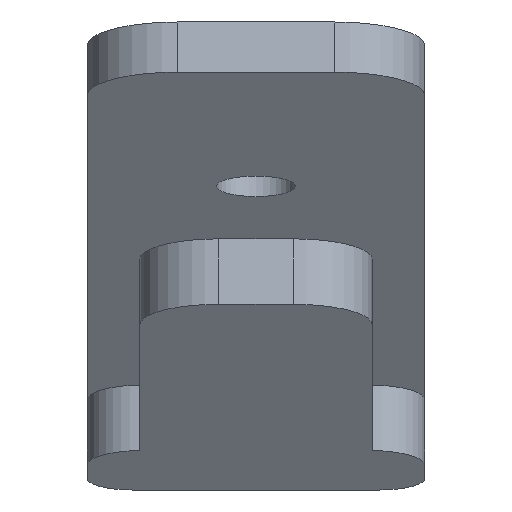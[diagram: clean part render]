
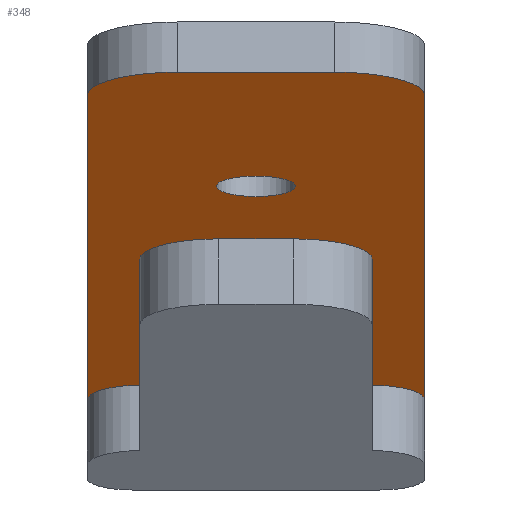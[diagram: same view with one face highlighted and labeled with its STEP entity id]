
A CAD part, left-side view. The second image highlights one B-rep face of the part: STEP entity #348.
In plain terms, the highlighted planar face has unit normal (-0.259, 0, -0.966).
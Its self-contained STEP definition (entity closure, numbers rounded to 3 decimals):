
#15=FACE_BOUND('',#48,.T.);
#17=PLANE('',#383);
#28=FACE_OUTER_BOUND('',#47,.T.);
#47=EDGE_LOOP('',(#240,#241,#242,#243,#244,#245,#246,#247,#248,#249,#250,
#251));
#48=EDGE_LOOP('',(#252));
#68=LINE('',#536,#101);
#69=LINE('',#540,#102);
#70=LINE('',#544,#103);
#71=LINE('',#548,#104);
#72=LINE('',#552,#105);
#73=LINE('',#556,#106);
#101=VECTOR('',#428,10.);
#102=VECTOR('',#431,10.);
#103=VECTOR('',#434,10.);
#104=VECTOR('',#437,10.);
#105=VECTOR('',#440,10.);
#106=VECTOR('',#443,10.);
#134=CIRCLE('',#382,1.75);
#135=CIRCLE('',#384,4.);
#136=CIRCLE('',#385,4.);
#137=CIRCLE('',#386,2.5);
#138=CIRCLE('',#387,3.5);
#139=CIRCLE('',#388,3.5);
#140=CIRCLE('',#389,2.5);
#152=VERTEX_POINT('',#530);
#153=VERTEX_POINT('',#534);
#154=VERTEX_POINT('',#535);
#155=VERTEX_POINT('',#537);
#156=VERTEX_POINT('',#539);
#157=VERTEX_POINT('',#541);
#158=VERTEX_POINT('',#543);
#159=VERTEX_POINT('',#545);
#160=VERTEX_POINT('',#547);
#161=VERTEX_POINT('',#549);
#162=VERTEX_POINT('',#551);
#163=VERTEX_POINT('',#553);
#164=VERTEX_POINT('',#555);
#187=EDGE_CURVE('',#152,#152,#134,.T.);
#188=EDGE_CURVE('',#153,#154,#68,.T.);
#189=EDGE_CURVE('',#154,#155,#135,.T.);
#190=EDGE_CURVE('',#155,#156,#69,.T.);
#191=EDGE_CURVE('',#156,#157,#136,.T.);
#192=EDGE_CURVE('',#157,#158,#70,.T.);
#193=EDGE_CURVE('',#159,#158,#137,.T.);
#194=EDGE_CURVE('',#160,#159,#71,.T.);
#195=EDGE_CURVE('',#161,#160,#138,.T.);
#196=EDGE_CURVE('',#162,#161,#72,.T.);
#197=EDGE_CURVE('',#163,#162,#139,.T.);
#198=EDGE_CURVE('',#164,#163,#73,.T.);
#199=EDGE_CURVE('',#153,#164,#140,.T.);
#240=ORIENTED_EDGE('',*,*,#188,.T.);
#241=ORIENTED_EDGE('',*,*,#189,.T.);
#242=ORIENTED_EDGE('',*,*,#190,.T.);
#243=ORIENTED_EDGE('',*,*,#191,.T.);
#244=ORIENTED_EDGE('',*,*,#192,.T.);
#245=ORIENTED_EDGE('',*,*,#193,.F.);
#246=ORIENTED_EDGE('',*,*,#194,.F.);
#247=ORIENTED_EDGE('',*,*,#195,.F.);
#248=ORIENTED_EDGE('',*,*,#196,.F.);
#249=ORIENTED_EDGE('',*,*,#197,.F.);
#250=ORIENTED_EDGE('',*,*,#198,.F.);
#251=ORIENTED_EDGE('',*,*,#199,.F.);
#252=ORIENTED_EDGE('',*,*,#187,.F.);
#348=ADVANCED_FACE('',(#28,#15),#17,.T.);
#382=AXIS2_PLACEMENT_3D('',#532,#424,#425);
#383=AXIS2_PLACEMENT_3D('',#533,#426,#427);
#384=AXIS2_PLACEMENT_3D('',#538,#429,#430);
#385=AXIS2_PLACEMENT_3D('',#542,#432,#433);
#386=AXIS2_PLACEMENT_3D('',#546,#435,#436);
#387=AXIS2_PLACEMENT_3D('',#550,#438,#439);
#388=AXIS2_PLACEMENT_3D('',#554,#441,#442);
#389=AXIS2_PLACEMENT_3D('',#557,#444,#445);
#424=DIRECTION('center_axis',(-0.259,0.,
-0.966));
#425=DIRECTION('ref_axis',(0.,-1.,0.));
#426=DIRECTION('center_axis',(-0.259,0.,
-0.966));
#427=DIRECTION('ref_axis',(0.,-1.,0.));
#428=DIRECTION('',(-0.966,0.,0.259));
#429=DIRECTION('center_axis',(-0.259,0.,
-0.966));
#430=DIRECTION('ref_axis',(0.,-1.,0.));
#431=DIRECTION('',(0.,1.,0.));
#432=DIRECTION('center_axis',(-0.259,0.,
-0.966));
#433=DIRECTION('ref_axis',(-0.966,0.,0.259));
#434=DIRECTION('',(0.966,0.,-0.259));
#435=DIRECTION('center_axis',(-0.259,0.,
-0.966));
#436=DIRECTION('ref_axis',(-0.964,0.07,0.258));
#437=DIRECTION('',(0.966,0.,-0.259));
#438=DIRECTION('center_axis',(-0.259,0.,
-0.966));
#439=DIRECTION('ref_axis',(-0.683,0.707,0.183));
#440=DIRECTION('',(0.,1.,0.));
#441=DIRECTION('center_axis',(-0.259,0.,
-0.966));
#442=DIRECTION('ref_axis',(-0.683,-0.707,0.183));
#443=DIRECTION('',(-0.966,0.,0.259));
#444=DIRECTION('center_axis',(-0.259,0.,
-0.966));
#445=DIRECTION('ref_axis',(-0.964,-0.07,0.258));
#530=CARTESIAN_POINT('',(845.807,-15.002,-151.431));
#532=CARTESIAN_POINT('Origin',(845.807,-16.752,-151.431));
#533=CARTESIAN_POINT('Origin',(854.006,-16.752,-153.627));
#534=CARTESIAN_POINT('',(881.048,-24.227,-160.874));
#535=CARTESIAN_POINT('',(830.827,-24.227,-147.417));
#536=CARTESIAN_POINT('',(881.048,-24.227,-160.874));
#537=CARTESIAN_POINT('',(826.963,-20.227,-146.381));
#538=CARTESIAN_POINT('Origin',(830.827,-20.227,-147.417));
#539=CARTESIAN_POINT('',(826.963,-13.277,-146.381));
#540=CARTESIAN_POINT('',(826.963,-20.227,-146.381));
#541=CARTESIAN_POINT('',(830.827,-9.277,-147.417));
#542=CARTESIAN_POINT('Origin',(830.827,-13.277,-147.417));
#543=CARTESIAN_POINT('',(881.048,-9.277,-160.874));
#544=CARTESIAN_POINT('',(830.827,-9.277,-147.417));
#545=CARTESIAN_POINT('',(878.64,-11.602,-160.228));
#546=CARTESIAN_POINT('Origin',(881.048,-11.777,-160.874));
#547=CARTESIAN_POINT('',(857.873,-11.602,-154.664));
#548=CARTESIAN_POINT('',(866.323,-11.602,-156.928));
#549=CARTESIAN_POINT('',(854.492,-15.102,-153.758));
#550=CARTESIAN_POINT('Origin',(857.873,-15.102,-154.664));
#551=CARTESIAN_POINT('',(854.492,-18.402,-153.758));
#552=CARTESIAN_POINT('',(854.492,-17.752,-153.758));
#553=CARTESIAN_POINT('',(857.873,-21.902,-154.664));
#554=CARTESIAN_POINT('Origin',(857.873,-18.402,-154.664));
#555=CARTESIAN_POINT('',(878.64,-21.902,-160.228));
#556=CARTESIAN_POINT('',(866.323,-21.902,-156.928));
#557=CARTESIAN_POINT('Origin',(881.048,-21.727,-160.874));
